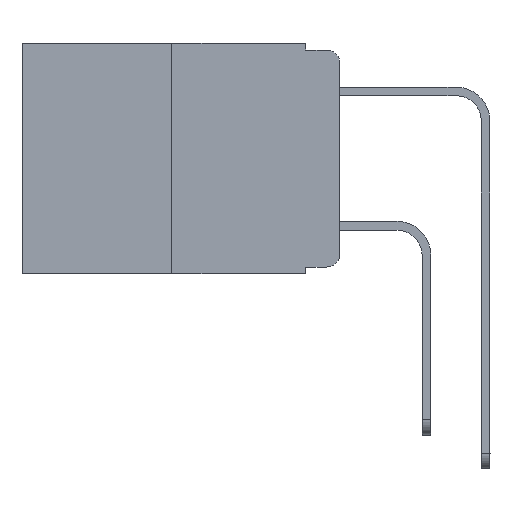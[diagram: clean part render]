
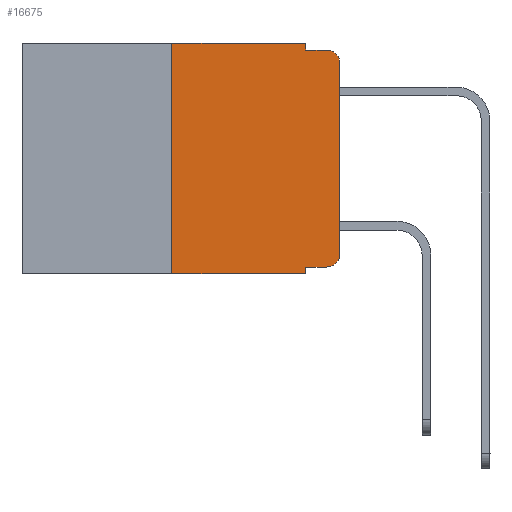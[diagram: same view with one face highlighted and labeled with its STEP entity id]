
A CAD part, left-side view. The second image highlights one B-rep face of the part: STEP entity #16675.
In plain terms, the highlighted planar face has unit normal (-1, 0, 0).
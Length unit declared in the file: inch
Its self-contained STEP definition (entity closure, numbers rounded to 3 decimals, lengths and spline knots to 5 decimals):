
#24 = CARTESIAN_POINT ( 'NONE',  ( 0., 0.25, -0.343 ) ) ;
#171 = EDGE_CURVE ( 'NONE', #20978, #21596, #22202, .T. ) ;
#703 = PLANE ( 'NONE',  #21982 ) ;
#713 = LINE ( 'NONE', #11592, #3975 ) ;
#894 = EDGE_CURVE ( 'NONE', #16767, #6571, #8932, .T. ) ;
#936 = AXIS2_PLACEMENT_3D ( 'NONE', #23057, #21065, #11917 ) ;
#1265 = EDGE_CURVE ( 'NONE', #5070, #7215, #22389, .T. ) ;
#1320 = ORIENTED_EDGE ( 'NONE', *, *, #3581, .F. ) ;
#1348 = VECTOR ( 'NONE', #20744, 39.37008 ) ;
#1457 = ORIENTED_EDGE ( 'NONE', *, *, #20391, .F. ) ;
#1820 = EDGE_CURVE ( 'NONE', #7215, #16767, #15143, .T. ) ;
#2063 = DIRECTION ( 'NONE',  ( 0., 0., -1. ) ) ;
#2529 = ORIENTED_EDGE ( 'NONE', *, *, #2658, .F. ) ;
#2658 = EDGE_CURVE ( 'NONE', #20978, #3586, #713, .T. ) ;
#2810 = DIRECTION ( 'NONE',  ( 1., 0., 0. ) ) ;
#2999 = DIRECTION ( 'NONE',  ( 0., -1., 0. ) ) ;
#3034 = CARTESIAN_POINT ( 'NONE',  ( 0., 0.051, 0. ) ) ;
#3260 = ORIENTED_EDGE ( 'NONE', *, *, #171, .T. ) ;
#3275 = AXIS2_PLACEMENT_3D ( 'NONE', #9207, #11293, #2063 ) ;
#3581 = EDGE_CURVE ( 'NONE', #16168, #5550, #8386, .T. ) ;
#3586 = VERTEX_POINT ( 'NONE', #20800 ) ;
#3727 = ORIENTED_EDGE ( 'NONE', *, *, #22183, .F. ) ;
#3975 = VECTOR ( 'NONE', #6546, 39.37008 ) ;
#4004 = CIRCLE ( 'NONE', #3275, 0.02 ) ;
#4805 = ORIENTED_EDGE ( 'NONE', *, *, #1265, .T. ) ;
#4846 = DIRECTION ( 'NONE',  ( 0., 0., 1. ) ) ;
#5070 = VERTEX_POINT ( 'NONE', #16615 ) ;
#5296 = VECTOR ( 'NONE', #13034, 39.37008 ) ;
#5550 = VERTEX_POINT ( 'NONE', #16469 ) ;
#6090 = FACE_OUTER_BOUND ( 'NONE', #9588, .T. ) ;
#6546 = DIRECTION ( 'NONE',  ( 0., 0., 1. ) ) ;
#6571 = VERTEX_POINT ( 'NONE', #20615 ) ;
#6606 = CARTESIAN_POINT ( 'NONE',  ( 0., 0.051, -0.01 ) ) ;
#6703 = LINE ( 'NONE', #21242, #10800 ) ;
#7048 = CARTESIAN_POINT ( 'NONE',  ( 0., 0., 0. ) ) ;
#7215 = VERTEX_POINT ( 'NONE', #16555 ) ;
#8386 = LINE ( 'NONE', #6606, #18265 ) ;
#8566 = EDGE_CURVE ( 'NONE', #6571, #5550, #4004, .T. ) ;
#8932 = LINE ( 'NONE', #7048, #22677 ) ;
#9207 = CARTESIAN_POINT ( 'NONE',  ( 0., 0.02, -0.03 ) ) ;
#9538 = CARTESIAN_POINT ( 'NONE',  ( 0., 0.473, -0.343 ) ) ;
#9588 = EDGE_LOOP ( 'NONE', ( #14239, #16175, #1320, #3727, #1457, #2529, #3260, #10399, #4805, #13355 ) ) ;
#9610 = CARTESIAN_POINT ( 'NONE',  ( 0., 0.051, -0.333 ) ) ;
#9950 = DIRECTION ( 'NONE',  ( 0., 0., -1. ) ) ;
#10227 = DIRECTION ( 'NONE',  ( 0., 0., -1. ) ) ;
#10399 = ORIENTED_EDGE ( 'NONE', *, *, #19576, .F. ) ;
#10800 = VECTOR ( 'NONE', #10227, 39.37008 ) ;
#11293 = DIRECTION ( 'NONE',  ( -1., 0., 0. ) ) ;
#11592 = CARTESIAN_POINT ( 'NONE',  ( 0., 0.25, 0. ) ) ;
#11917 = DIRECTION ( 'NONE',  ( 0., 0., -1. ) ) ;
#11967 = CARTESIAN_POINT ( 'NONE',  ( 0., 0.051, -0.01 ) ) ;
#13034 = DIRECTION ( 'NONE',  ( 0., -1., 0. ) ) ;
#13355 = ORIENTED_EDGE ( 'NONE', *, *, #1820, .T. ) ;
#14239 = ORIENTED_EDGE ( 'NONE', *, *, #894, .T. ) ;
#14925 = VECTOR ( 'NONE', #15444, 39.37008 ) ;
#15097 = CARTESIAN_POINT ( 'NONE',  ( 0., 0.473, 0. ) ) ;
#15143 = CIRCLE ( 'NONE', #936, 0.02 ) ;
#15444 = DIRECTION ( 'NONE',  ( 0., -1., 0. ) ) ;
#15689 = CARTESIAN_POINT ( 'NONE',  ( 0., 0., -0.313 ) ) ;
#15797 = LINE ( 'NONE', #3034, #22126 ) ;
#16168 = VERTEX_POINT ( 'NONE', #11967 ) ;
#16175 = ORIENTED_EDGE ( 'NONE', *, *, #8566, .T. ) ;
#16469 = CARTESIAN_POINT ( 'NONE',  ( 0., 0.02, -0.01 ) ) ;
#16555 = CARTESIAN_POINT ( 'NONE',  ( 0., 0.02, -0.333 ) ) ;
#16615 = CARTESIAN_POINT ( 'NONE',  ( 0., 0.051, -0.333 ) ) ;
#16675 = ADVANCED_FACE ( 'NONE', ( #6090 ), #703, .F. ) ;
#16767 = VERTEX_POINT ( 'NONE', #15689 ) ;
#17082 = LINE ( 'NONE', #18866, #14925 ) ;
#18265 = VECTOR ( 'NONE', #2999, 39.37008 ) ;
#18866 = CARTESIAN_POINT ( 'NONE',  ( 0., 0.473, 0. ) ) ;
#19215 = DIRECTION ( 'NONE',  ( 0., 0., -1. ) ) ;
#19576 = EDGE_CURVE ( 'NONE', #5070, #21596, #6703, .T. ) ;
#20391 = EDGE_CURVE ( 'NONE', #3586, #21614, #17082, .T. ) ;
#20615 = CARTESIAN_POINT ( 'NONE',  ( 0., 0., -0.03 ) ) ;
#20744 = DIRECTION ( 'NONE',  ( 0., -1., 0. ) ) ;
#20800 = CARTESIAN_POINT ( 'NONE',  ( 0., 0.25, 0. ) ) ;
#20978 = VERTEX_POINT ( 'NONE', #24 ) ;
#21065 = DIRECTION ( 'NONE',  ( -1., 0., 0. ) ) ;
#21242 = CARTESIAN_POINT ( 'NONE',  ( 0., 0.051, 0. ) ) ;
#21596 = VERTEX_POINT ( 'NONE', #21944 ) ;
#21614 = VERTEX_POINT ( 'NONE', #21697 ) ;
#21697 = CARTESIAN_POINT ( 'NONE',  ( 0., 0.051, 0. ) ) ;
#21944 = CARTESIAN_POINT ( 'NONE',  ( 0., 0.051, -0.343 ) ) ;
#21982 = AXIS2_PLACEMENT_3D ( 'NONE', #15097, #2810, #9950 ) ;
#22126 = VECTOR ( 'NONE', #19215, 39.37008 ) ;
#22183 = EDGE_CURVE ( 'NONE', #21614, #16168, #15797, .T. ) ;
#22202 = LINE ( 'NONE', #9538, #5296 ) ;
#22389 = LINE ( 'NONE', #9610, #1348 ) ;
#22677 = VECTOR ( 'NONE', #4846, 39.37008 ) ;
#23057 = CARTESIAN_POINT ( 'NONE',  ( 0., 0.02, -0.313 ) ) ;
